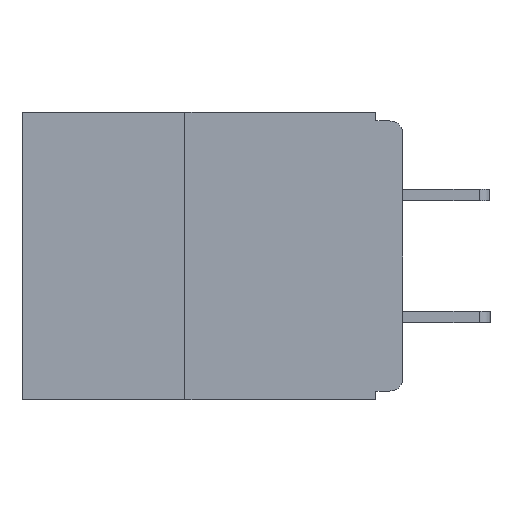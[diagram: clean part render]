
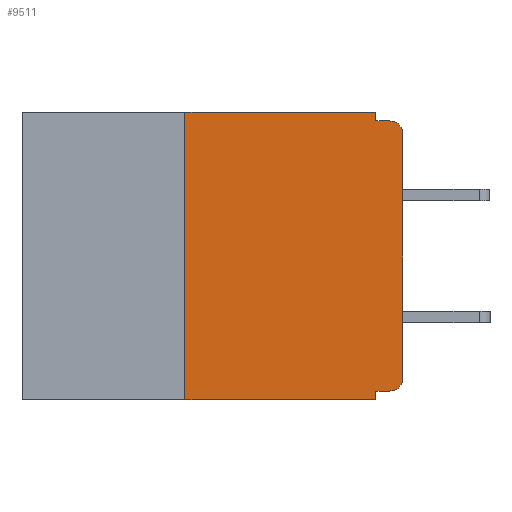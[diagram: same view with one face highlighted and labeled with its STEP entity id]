
A CAD part, left-side view. The second image highlights one B-rep face of the part: STEP entity #9511.
In plain terms, the highlighted planar face has unit normal (-1, 0, 0).
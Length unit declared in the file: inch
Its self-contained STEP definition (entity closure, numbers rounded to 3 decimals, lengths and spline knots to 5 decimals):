
#104 = ORIENTED_EDGE ( 'NONE', *, *, #10860, .T. ) ;
#235 = VERTEX_POINT ( 'NONE', #18431 ) ;
#396 = DIRECTION ( 'NONE',  ( 0., 1., 0. ) ) ;
#466 = EDGE_CURVE ( 'NONE', #235, #9940, #16431, .T. ) ;
#617 = VERTEX_POINT ( 'NONE', #6417 ) ;
#619 = EDGE_CURVE ( 'NONE', #13831, #617, #14260, .T. ) ;
#793 = ORIENTED_EDGE ( 'NONE', *, *, #9275, .T. ) ;
#880 = VECTOR ( 'NONE', #13769, 39.37008 ) ;
#882 = ORIENTED_EDGE ( 'NONE', *, *, #619, .F. ) ;
#1052 = CIRCLE ( 'NONE', #9162, 0.015 ) ;
#1526 = ORIENTED_EDGE ( 'NONE', *, *, #3656, .F. ) ;
#1550 = EDGE_CURVE ( 'NONE', #13242, #9940, #11419, .T. ) ;
#1996 = CARTESIAN_POINT ( 'NONE',  ( 0., 0.031, -0.33 ) ) ;
#2000 = ORIENTED_EDGE ( 'NONE', *, *, #11669, .F. ) ;
#2621 = EDGE_CURVE ( 'NONE', #13242, #10706, #5117, .T. ) ;
#2623 = ORIENTED_EDGE ( 'NONE', *, *, #2621, .F. ) ;
#2968 = ORIENTED_EDGE ( 'NONE', *, *, #1550, .T. ) ;
#3002 = ORIENTED_EDGE ( 'NONE', *, *, #466, .F. ) ;
#3419 = VECTOR ( 'NONE', #9709, 39.37008 ) ;
#3528 = ORIENTED_EDGE ( 'NONE', *, *, #14028, .F. ) ;
#3535 = DIRECTION ( 'NONE',  ( 0., 0., -1. ) ) ;
#3561 = DIRECTION ( 'NONE',  ( -1., 0., 0. ) ) ;
#3569 = ORIENTED_EDGE ( 'NONE', *, *, #7312, .T. ) ;
#3583 = CARTESIAN_POINT ( 'NONE',  ( 0., 0.015, -0.305 ) ) ;
#3656 = EDGE_CURVE ( 'NONE', #17246, #13831, #11365, .T. ) ;
#4021 = VERTEX_POINT ( 'NONE', #11819 ) ;
#4680 = CARTESIAN_POINT ( 'NONE',  ( 0., 0.437, 0. ) ) ;
#4892 = DIRECTION ( 'NONE',  ( 0., -1., 0. ) ) ;
#5117 = LINE ( 'NONE', #13248, #880 ) ;
#5495 = VERTEX_POINT ( 'NONE', #14747 ) ;
#5833 = DIRECTION ( 'NONE',  ( 0., 0., -1. ) ) ;
#5868 = VECTOR ( 'NONE', #4892, 39.37008 ) ;
#5926 = DIRECTION ( 'NONE',  ( 0., 0., 1. ) ) ;
#6129 = CARTESIAN_POINT ( 'NONE',  ( 0., 0.25, -0.33 ) ) ;
#6179 = CARTESIAN_POINT ( 'NONE',  ( 0., 0.031, -0.01 ) ) ;
#6335 = LINE ( 'NONE', #4680, #5868 ) ;
#6349 = CARTESIAN_POINT ( 'NONE',  ( 0., 0.031, -0.33 ) ) ;
#6417 = CARTESIAN_POINT ( 'NONE',  ( 0., 0.015, -0.01 ) ) ;
#7146 = EDGE_LOOP ( 'NONE', ( #104, #793, #882, #1526, #2000, #2623, #2968, #3002, #3528, #3569 ) ) ;
#7149 = CARTESIAN_POINT ( 'NONE',  ( 0., 0.031, 0. ) ) ;
#7312 = EDGE_CURVE ( 'NONE', #18760, #4021, #1052, .T. ) ;
#7474 = VECTOR ( 'NONE', #5833, 39.37008 ) ;
#8668 = DIRECTION ( 'NONE',  ( 0., -1., 0. ) ) ;
#9162 = AXIS2_PLACEMENT_3D ( 'NONE', #3583, #3561, #3535 ) ;
#9275 = EDGE_CURVE ( 'NONE', #5495, #617, #13192, .T. ) ;
#9288 = CARTESIAN_POINT ( 'NONE',  ( 0., 0., -0.01 ) ) ;
#9511 = ADVANCED_FACE ( 'NONE', ( #10065 ), #10592, .F. ) ;
#9709 = DIRECTION ( 'NONE',  ( 0., -1., 0. ) ) ;
#9940 = VERTEX_POINT ( 'NONE', #6349 ) ;
#10015 = CARTESIAN_POINT ( 'NONE',  ( 0., 0.031, 0. ) ) ;
#10065 = FACE_OUTER_BOUND ( 'NONE', #7146, .T. ) ;
#10073 = CARTESIAN_POINT ( 'NONE',  ( 0., 0., 0. ) ) ;
#10080 = VECTOR ( 'NONE', #8668, 39.37008 ) ;
#10469 = DIRECTION ( 'NONE',  ( 0., 0., -1. ) ) ;
#10484 = DIRECTION ( 'NONE',  ( 1., 0., 0. ) ) ;
#10537 = CARTESIAN_POINT ( 'NONE',  ( 0., 0.437, 0. ) ) ;
#10592 = PLANE ( 'NONE',  #16150 ) ;
#10706 = VERTEX_POINT ( 'NONE', #18547 ) ;
#10860 = EDGE_CURVE ( 'NONE', #4021, #5495, #16395, .T. ) ;
#11054 = CARTESIAN_POINT ( 'NONE',  ( 0., 0.015, -0.32 ) ) ;
#11365 = LINE ( 'NONE', #10015, #7474 ) ;
#11419 = LINE ( 'NONE', #15614, #3419 ) ;
#11669 = EDGE_CURVE ( 'NONE', #10706, #17246, #6335, .T. ) ;
#11819 = CARTESIAN_POINT ( 'NONE',  ( 0., 0., -0.305 ) ) ;
#12460 = DIRECTION ( 'NONE',  ( 0., 0., -1. ) ) ;
#12480 = DIRECTION ( 'NONE',  ( -1., 0., 0. ) ) ;
#12503 = CARTESIAN_POINT ( 'NONE',  ( 0., 0.015, -0.025 ) ) ;
#12780 = VECTOR ( 'NONE', #17081, 39.37008 ) ;
#13192 = CIRCLE ( 'NONE', #15544, 0.015 ) ;
#13242 = VERTEX_POINT ( 'NONE', #6129 ) ;
#13248 = CARTESIAN_POINT ( 'NONE',  ( 0., 0.25, -0.33 ) ) ;
#13297 = VECTOR ( 'NONE', #396, 39.37008 ) ;
#13769 = DIRECTION ( 'NONE',  ( 0., 0., 1. ) ) ;
#13831 = VERTEX_POINT ( 'NONE', #6179 ) ;
#13901 = CARTESIAN_POINT ( 'NONE',  ( 0., 0., -0.32 ) ) ;
#14028 = EDGE_CURVE ( 'NONE', #18760, #235, #16533, .T. ) ;
#14260 = LINE ( 'NONE', #9288, #10080 ) ;
#14747 = CARTESIAN_POINT ( 'NONE',  ( 0., 0., -0.025 ) ) ;
#15491 = VECTOR ( 'NONE', #5926, 39.37008 ) ;
#15544 = AXIS2_PLACEMENT_3D ( 'NONE', #12503, #12480, #12460 ) ;
#15614 = CARTESIAN_POINT ( 'NONE',  ( 0., 0.437, -0.33 ) ) ;
#16150 = AXIS2_PLACEMENT_3D ( 'NONE', #10537, #10484, #10469 ) ;
#16395 = LINE ( 'NONE', #10073, #15491 ) ;
#16431 = LINE ( 'NONE', #1996, #12780 ) ;
#16533 = LINE ( 'NONE', #13901, #13297 ) ;
#17081 = DIRECTION ( 'NONE',  ( 0., 0., -1. ) ) ;
#17246 = VERTEX_POINT ( 'NONE', #7149 ) ;
#18431 = CARTESIAN_POINT ( 'NONE',  ( 0., 0.031, -0.32 ) ) ;
#18547 = CARTESIAN_POINT ( 'NONE',  ( 0., 0.25, 0. ) ) ;
#18760 = VERTEX_POINT ( 'NONE', #11054 ) ;
